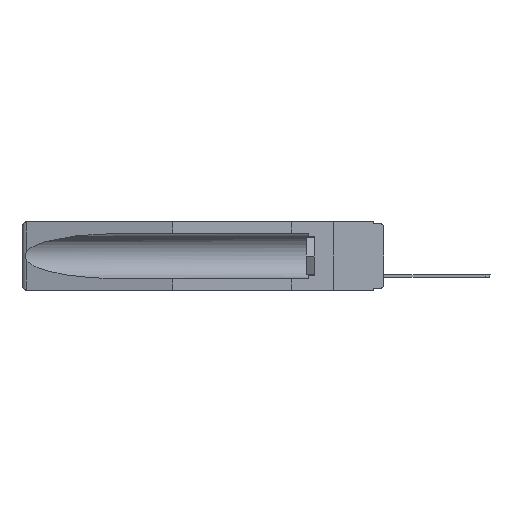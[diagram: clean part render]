
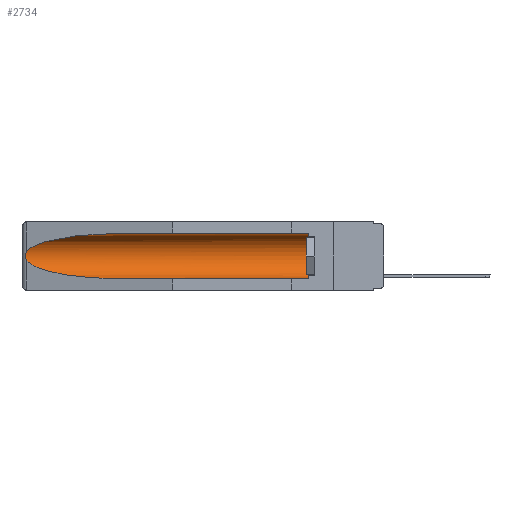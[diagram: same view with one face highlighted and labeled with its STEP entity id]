
A CAD part, left-side view. The second image highlights one B-rep face of the part: STEP entity #2734.
In plain terms, the highlighted cylindrical face has radius 2.857 mm (diameter 5.715 mm), a partial arc.
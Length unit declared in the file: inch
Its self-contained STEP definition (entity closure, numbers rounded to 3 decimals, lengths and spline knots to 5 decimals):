
#8 = CARTESIAN_POINT ( 'NONE',  ( 0.155, 0.126, -0.284 ) ) ;
#565 = AXIS2_PLACEMENT_3D ( 'NONE', #6379, #22292, #18486 ) ;
#649 = FACE_OUTER_BOUND ( 'NONE', #10236, .T. ) ;
#1568 = AXIS2_PLACEMENT_3D ( 'NONE', #18610, #8625, #2471 ) ;
#2176 = CARTESIAN_POINT ( 'NONE',  ( 0.26597, 1.52961, -0.15275 ) ) ;
#2471 = DIRECTION ( 'NONE',  ( 0., 0., 1. ) ) ;
#2612 = VERTEX_POINT ( 'NONE', #8 ) ;
#2734 = ADVANCED_FACE ( 'NONE', ( #649 ), #8088, .F. ) ;
#2852 = VERTEX_POINT ( 'NONE', #23214 ) ;
#4535 = CARTESIAN_POINT ( 'NONE',  ( 0.155, 1.07973, -0.059 ) ) ;
#4539 = CARTESIAN_POINT ( 'NONE',  ( 0.155, -0.30754, -0.284 ) ) ;
#4604 = CARTESIAN_POINT ( 'NONE',  ( 0.26537, 1.52718, -0.19328 ) ) ;
#4790 = DIRECTION ( 'NONE',  ( 0., 1., 0. ) ) ;
#5676 = ORIENTED_EDGE ( 'NONE', *, *, #18287, .T. ) ;
#5718 = B_SPLINE_CURVE_WITH_KNOTS ( 'NONE', 3,
 ( #17957, #2176, #10187, #23998, #13754, #18192, #14268, #16229, #20061, #17687 ),
 .UNSPECIFIED., .F., .F.,
 ( 4, 2, 2, 2, 4 ),
 ( 0., 0.00029, 0.00058, 0.00087, 0.00117 ),
 .UNSPECIFIED. ) ;
#6379 = CARTESIAN_POINT ( 'NONE',  ( 0.155, 0.126, -0.1715 ) ) ;
#6605 = CARTESIAN_POINT ( 'NONE',  ( 0.155, 1.07973, -0.284 ) ) ;
#6842 = CARTESIAN_POINT ( 'NONE',  ( 0.21114, 1.30732, -0.059 ) ) ;
#6995 = CARTESIAN_POINT ( 'NONE',  ( 0.155, 1.07973, -0.059 ) ) ;
#8088 = CYLINDRICAL_SURFACE ( 'NONE', #1568, 0.1125 ) ;
#8625 = DIRECTION ( 'NONE',  ( 0., 1., 0. ) ) ;
#9478 = VECTOR ( 'NONE', #4790, 39.37008 ) ;
#9604 = EDGE_CURVE ( 'NONE', #11484, #2852, #18751, .T. ) ;
#10187 = CARTESIAN_POINT ( 'NONE',  ( 0.26654, 1.53092, -0.15636 ) ) ;
#10236 = EDGE_LOOP ( 'NONE', ( #19791, #19787, #17863, #19196, #21728, #5676 ) ) ;
#11177 = VERTEX_POINT ( 'NONE', #22204 ) ;
#11484 = VERTEX_POINT ( 'NONE', #4535 ) ;
#11704 = DIRECTION ( 'NONE',  ( 0., 1., 0. ) ) ;
#12115 = EDGE_CURVE ( 'NONE', #24483, #25679, #17589, .T. ) ;
#13719 = CARTESIAN_POINT ( 'NONE',  ( 0.155, 1.07973, -0.284 ) ) ;
#13754 = CARTESIAN_POINT ( 'NONE',  ( 0.2675, 1.53308, -0.16763 ) ) ;
#14268 = CARTESIAN_POINT ( 'NONE',  ( 0.2673, 1.53269, -0.17917 ) ) ;
#14886 = CARTESIAN_POINT ( 'NONE',  ( 0.25451, 1.48313, -0.09465 ) ) ;
#16229 = CARTESIAN_POINT ( 'NONE',  ( 0.26655, 1.53094, -0.18657 ) ) ;
#17589 =( BOUNDED_CURVE ( )  B_SPLINE_CURVE ( 3, ( #21472, #25451, #21740, #13719 ),
 .UNSPECIFIED., .F., .T. ) 
 B_SPLINE_CURVE_WITH_KNOTS ( ( 4, 4 ),
 ( 0.1948, 1.5708 ),
 .UNSPECIFIED. ) 
 CURVE ( )  GEOMETRIC_REPRESENTATION_ITEM ( )  RATIONAL_B_SPLINE_CURVE ( ( 1., 0.848, 0.848, 1. ) ) 
 REPRESENTATION_ITEM ( '' )  );
#17610 = LINE ( 'NONE', #23663, #19119 ) ;
#17687 = CARTESIAN_POINT ( 'NONE',  ( 0.26537, 1.52718, -0.19328 ) ) ;
#17863 = ORIENTED_EDGE ( 'NONE', *, *, #12115, .T. ) ;
#17957 = CARTESIAN_POINT ( 'NONE',  ( 0.26537, 1.52718, -0.14972 ) ) ;
#18192 = CARTESIAN_POINT ( 'NONE',  ( 0.2675, 1.53308, -0.17534 ) ) ;
#18287 = EDGE_CURVE ( 'NONE', #11177, #11484, #17610, .T. ) ;
#18486 = DIRECTION ( 'NONE',  ( 0., 0., 1. ) ) ;
#18610 = CARTESIAN_POINT ( 'NONE',  ( 0.155, -0.30754, -0.1715 ) ) ;
#18751 =( BOUNDED_CURVE ( )  B_SPLINE_CURVE ( 3, ( #6995, #6842, #14886, #22891 ),
 .UNSPECIFIED., .F., .T. ) 
 B_SPLINE_CURVE_WITH_KNOTS ( ( 4, 4 ),
 ( 4.71239, 6.08839 ),
 .UNSPECIFIED. ) 
 CURVE ( )  GEOMETRIC_REPRESENTATION_ITEM ( )  RATIONAL_B_SPLINE_CURVE ( ( 1., 0.848, 0.848, 1. ) ) 
 REPRESENTATION_ITEM ( '' )  );
#18981 = EDGE_CURVE ( 'NONE', #2612, #25679, #20461, .T. ) ;
#19119 = VECTOR ( 'NONE', #11704, 39.37008 ) ;
#19196 = ORIENTED_EDGE ( 'NONE', *, *, #18981, .F. ) ;
#19787 = ORIENTED_EDGE ( 'NONE', *, *, #21356, .T. ) ;
#19791 = ORIENTED_EDGE ( 'NONE', *, *, #9604, .T. ) ;
#19866 = EDGE_CURVE ( 'NONE', #2612, #11177, #23205, .T. ) ;
#20061 = CARTESIAN_POINT ( 'NONE',  ( 0.26597, 1.5296, -0.19026 ) ) ;
#20461 = LINE ( 'NONE', #4539, #9478 ) ;
#21356 = EDGE_CURVE ( 'NONE', #2852, #24483, #5718, .T. ) ;
#21472 = CARTESIAN_POINT ( 'NONE',  ( 0.26537, 1.52718, -0.19328 ) ) ;
#21728 = ORIENTED_EDGE ( 'NONE', *, *, #19866, .T. ) ;
#21740 = CARTESIAN_POINT ( 'NONE',  ( 0.21114, 1.30732, -0.284 ) ) ;
#22204 = CARTESIAN_POINT ( 'NONE',  ( 0.155, 0.126, -0.059 ) ) ;
#22292 = DIRECTION ( 'NONE',  ( 0., -1., 0. ) ) ;
#22891 = CARTESIAN_POINT ( 'NONE',  ( 0.26537, 1.52718, -0.14972 ) ) ;
#23205 = CIRCLE ( 'NONE', #565, 0.1125 ) ;
#23214 = CARTESIAN_POINT ( 'NONE',  ( 0.26537, 1.52718, -0.14972 ) ) ;
#23663 = CARTESIAN_POINT ( 'NONE',  ( 0.155, -0.30754, -0.059 ) ) ;
#23998 = CARTESIAN_POINT ( 'NONE',  ( 0.2673, 1.5327, -0.16383 ) ) ;
#24483 = VERTEX_POINT ( 'NONE', #4604 ) ;
#25451 = CARTESIAN_POINT ( 'NONE',  ( 0.25451, 1.48313, -0.24835 ) ) ;
#25679 = VERTEX_POINT ( 'NONE', #6605 ) ;
